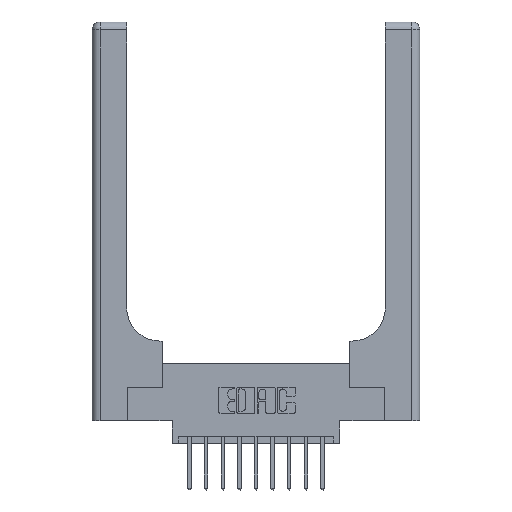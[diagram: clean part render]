
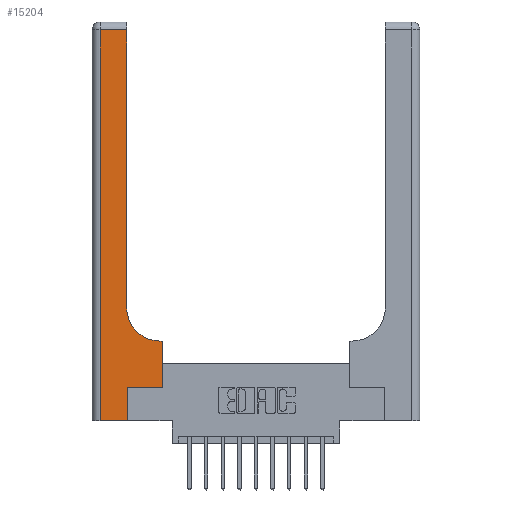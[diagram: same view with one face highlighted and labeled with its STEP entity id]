
A CAD part, top view. The second image highlights one B-rep face of the part: STEP entity #15204.
In plain terms, the highlighted planar face has unit normal (0, 0, 1).
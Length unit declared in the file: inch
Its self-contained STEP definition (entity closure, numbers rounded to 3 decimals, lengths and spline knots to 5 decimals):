
#54 = CARTESIAN_POINT ( 'NONE',  ( 0.26, 0.85, 0.37 ) ) ;
#85 = DIRECTION ( 'NONE',  ( 1., 0., 0. ) ) ;
#107 = EDGE_CURVE ( 'NONE', #7165, #166, #3863, .T. ) ;
#166 = VERTEX_POINT ( 'NONE', #4171 ) ;
#189 = DIRECTION ( 'NONE',  ( 0., -1., 0. ) ) ;
#206 = EDGE_CURVE ( 'NONE', #166, #14675, #4400, .T. ) ;
#262 = CARTESIAN_POINT ( 'NONE',  ( 0., 3., 0.37 ) ) ;
#440 = CARTESIAN_POINT ( 'NONE',  ( 0., 2.94, 0.37 ) ) ;
#594 = LINE ( 'NONE', #2051, #5943 ) ;
#995 = VECTOR ( 'NONE', #12723, 39.37008 ) ;
#1494 = VECTOR ( 'NONE', #189, 39.37008 ) ;
#1666 = LINE ( 'NONE', #440, #11152 ) ;
#1718 = VERTEX_POINT ( 'NONE', #14342 ) ;
#1927 = ORIENTED_EDGE ( 'NONE', *, *, #13893, .T. ) ;
#2043 = VERTEX_POINT ( 'NONE', #54 ) ;
#2051 = CARTESIAN_POINT ( 'NONE',  ( 0.26, 3., 0.37 ) ) ;
#2240 = ORIENTED_EDGE ( 'NONE', *, *, #11026, .T. ) ;
#2862 = EDGE_CURVE ( 'NONE', #14675, #2043, #12406, .T. ) ;
#3189 = CARTESIAN_POINT ( 'NONE',  ( 0.265, 0., 0.37 ) ) ;
#3227 = CARTESIAN_POINT ( 'NONE',  ( 0.51, 0.85, 0.37 ) ) ;
#3505 = VERTEX_POINT ( 'NONE', #7510 ) ;
#3634 = DIRECTION ( 'NONE',  ( 0., 1., 0. ) ) ;
#3863 = LINE ( 'NONE', #6369, #9902 ) ;
#3871 = LINE ( 'NONE', #3950, #4194 ) ;
#3950 = CARTESIAN_POINT ( 'NONE',  ( 0.265, 0., 0.37 ) ) ;
#3976 = DIRECTION ( 'NONE',  ( 0., 0., -1. ) ) ;
#4171 = CARTESIAN_POINT ( 'NONE',  ( 0.528, 0.6, 0.37 ) ) ;
#4194 = VECTOR ( 'NONE', #3634, 39.37008 ) ;
#4367 = ORIENTED_EDGE ( 'NONE', *, *, #13224, .T. ) ;
#4400 = LINE ( 'NONE', #15510, #10637 ) ;
#4789 = VERTEX_POINT ( 'NONE', #7898 ) ;
#5176 = EDGE_CURVE ( 'NONE', #10807, #1718, #1666, .T. ) ;
#5298 = ORIENTED_EDGE ( 'NONE', *, *, #2862, .T. ) ;
#5305 = DIRECTION ( 'NONE',  ( 0., 1., 0. ) ) ;
#5368 = DIRECTION ( 'NONE',  ( -1., 0., 0. ) ) ;
#5583 = ORIENTED_EDGE ( 'NONE', *, *, #11680, .T. ) ;
#5943 = VECTOR ( 'NONE', #6991, 39.37008 ) ;
#6341 = LINE ( 'NONE', #13695, #1494 ) ;
#6369 = CARTESIAN_POINT ( 'NONE',  ( 0.528, 0.25, 0.37 ) ) ;
#6404 = FACE_OUTER_BOUND ( 'NONE', #12038, .T. ) ;
#6991 = DIRECTION ( 'NONE',  ( 0., 1., 0. ) ) ;
#7165 = VERTEX_POINT ( 'NONE', #7472 ) ;
#7306 = ORIENTED_EDGE ( 'NONE', *, *, #206, .T. ) ;
#7472 = CARTESIAN_POINT ( 'NONE',  ( 0.528, 0.25, 0.37 ) ) ;
#7510 = CARTESIAN_POINT ( 'NONE',  ( 0.265, 0.25, 0.37 ) ) ;
#7643 = ORIENTED_EDGE ( 'NONE', *, *, #5176, .T. ) ;
#7732 = CARTESIAN_POINT ( 'NONE',  ( 0., 0., 0.37 ) ) ;
#7898 = CARTESIAN_POINT ( 'NONE',  ( 0.06, 0., 0.37 ) ) ;
#8117 = VERTEX_POINT ( 'NONE', #3189 ) ;
#8313 = AXIS2_PLACEMENT_3D ( 'NONE', #262, #3976, #11617 ) ;
#8374 = ORIENTED_EDGE ( 'NONE', *, *, #107, .T. ) ;
#8539 = CARTESIAN_POINT ( 'NONE',  ( 0.265, 0.25, 0.37 ) ) ;
#8889 = LINE ( 'NONE', #7732, #995 ) ;
#9516 = DIRECTION ( 'NONE',  ( 1., 0., 0. ) ) ;
#9902 = VECTOR ( 'NONE', #5305, 39.37008 ) ;
#10637 = VECTOR ( 'NONE', #13054, 39.37008 ) ;
#10807 = VERTEX_POINT ( 'NONE', #11886 ) ;
#11026 = EDGE_CURVE ( 'NONE', #1718, #4789, #6341, .T. ) ;
#11152 = VECTOR ( 'NONE', #5368, 39.37008 ) ;
#11463 = PLANE ( 'NONE',  #8313 ) ;
#11617 = DIRECTION ( 'NONE',  ( -1., 0., 0. ) ) ;
#11634 = VECTOR ( 'NONE', #9516, 39.37008 ) ;
#11680 = EDGE_CURVE ( 'NONE', #4789, #8117, #8889, .T. ) ;
#11886 = CARTESIAN_POINT ( 'NONE',  ( 0.26, 2.94, 0.37 ) ) ;
#11987 = EDGE_CURVE ( 'NONE', #3505, #7165, #13544, .T. ) ;
#12038 = EDGE_LOOP ( 'NONE', ( #1927, #7643, #2240, #5583, #4367, #13699, #8374, #7306, #5298 ) ) ;
#12406 = CIRCLE ( 'NONE', #14759, 0.25 ) ;
#12723 = DIRECTION ( 'NONE',  ( 1., 0., 0. ) ) ;
#13054 = DIRECTION ( 'NONE',  ( -1., 0., 0. ) ) ;
#13224 = EDGE_CURVE ( 'NONE', #8117, #3505, #3871, .T. ) ;
#13506 = DIRECTION ( 'NONE',  ( 0., 0., -1. ) ) ;
#13544 = LINE ( 'NONE', #8539, #11634 ) ;
#13635 = CARTESIAN_POINT ( 'NONE',  ( 0.51, 0.6, 0.37 ) ) ;
#13695 = CARTESIAN_POINT ( 'NONE',  ( 0.06, 3., 0.37 ) ) ;
#13699 = ORIENTED_EDGE ( 'NONE', *, *, #11987, .T. ) ;
#13893 = EDGE_CURVE ( 'NONE', #2043, #10807, #594, .T. ) ;
#14342 = CARTESIAN_POINT ( 'NONE',  ( 0.06, 2.94, 0.37 ) ) ;
#14675 = VERTEX_POINT ( 'NONE', #13635 ) ;
#14759 = AXIS2_PLACEMENT_3D ( 'NONE', #3227, #13506, #85 ) ;
#15204 = ADVANCED_FACE ( 'NONE', ( #6404 ), #11463, .F. ) ;
#15510 = CARTESIAN_POINT ( 'NONE',  ( 0.26, 0.6, 0.37 ) ) ;
